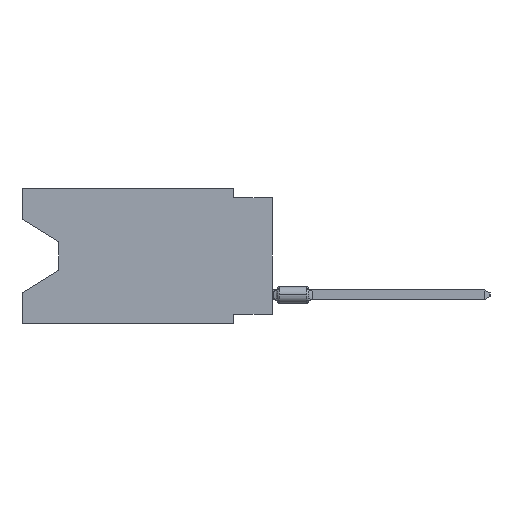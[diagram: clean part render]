
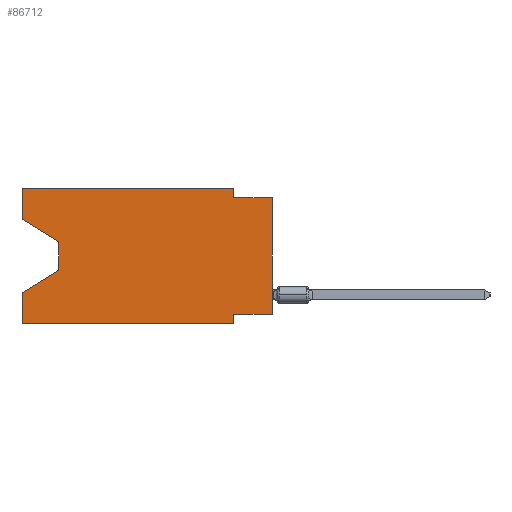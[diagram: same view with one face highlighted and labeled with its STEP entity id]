
A CAD part, left-side view. The second image highlights one B-rep face of the part: STEP entity #86712.
In plain terms, the highlighted planar face has unit normal (-1, 0, 0).
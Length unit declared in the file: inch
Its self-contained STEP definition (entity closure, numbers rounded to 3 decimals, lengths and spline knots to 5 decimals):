
#59 = DIRECTION ( 'NONE',  ( 0., 0., -1. ) ) ;
#190 = EDGE_CURVE ( 'NONE', #42665, #22390, #9721, .T. ) ;
#975 = DIRECTION ( 'NONE',  ( 0., -1., 0. ) ) ;
#1754 = DIRECTION ( 'NONE',  ( 0., 0., -1. ) ) ;
#4602 = VERTEX_POINT ( 'NONE', #24832 ) ;
#4651 = DIRECTION ( 'NONE',  ( 0., 0., 1. ) ) ;
#4712 = LINE ( 'NONE', #54291, #21248 ) ;
#5526 = EDGE_CURVE ( 'NONE', #4602, #62011, #58702, .T. ) ;
#5582 = LINE ( 'NONE', #12265, #63702 ) ;
#7689 = ORIENTED_EDGE ( 'NONE', *, *, #39928, .T. ) ;
#7878 = EDGE_LOOP ( 'NONE', ( #89855, #53086, #50535, #82369, #21418, #40404, #60067, #7689, #98472, #72064, #13869, #52340 ) ) ;
#8539 = CARTESIAN_POINT ( 'NONE',  ( 0., 0.645, -0.08025 ) ) ;
#9721 = LINE ( 'NONE', #57287, #65462 ) ;
#10214 = DIRECTION ( 'NONE',  ( 0., 0., 1. ) ) ;
#10752 = CARTESIAN_POINT ( 'NONE',  ( 0., 0.645, -0.08025 ) ) ;
#11148 = VECTOR ( 'NONE', #1754, 39.37008 ) ;
#11389 = EDGE_CURVE ( 'NONE', #88643, #62011, #37881, .T. ) ;
#12265 = CARTESIAN_POINT ( 'NONE',  ( 0., 0.645, -0.35 ) ) ;
#13869 = ORIENTED_EDGE ( 'NONE', *, *, #35759, .F. ) ;
#16514 = CARTESIAN_POINT ( 'NONE',  ( 0., 0., -0.325 ) ) ;
#16777 = VECTOR ( 'NONE', #67468, 39.37008 ) ;
#16951 = CARTESIAN_POINT ( 'NONE',  ( 0., 0., -0.025 ) ) ;
#17165 = CARTESIAN_POINT ( 'NONE',  ( 0., 0.55, -0.138 ) ) ;
#18615 = DIRECTION ( 'NONE',  ( 0., -1., 0. ) ) ;
#19096 = DIRECTION ( 'NONE',  ( 0., 0., -1. ) ) ;
#20589 = PLANE ( 'NONE',  #83614 ) ;
#21248 = VECTOR ( 'NONE', #59, 39.37008 ) ;
#21418 = ORIENTED_EDGE ( 'NONE', *, *, #82533, .T. ) ;
#22390 = VERTEX_POINT ( 'NONE', #92120 ) ;
#22966 = CARTESIAN_POINT ( 'NONE',  ( 0., 0.645, -0.35 ) ) ;
#23075 = VERTEX_POINT ( 'NONE', #59653 ) ;
#23922 = VECTOR ( 'NONE', #71784, 39.37008 ) ;
#24470 = VECTOR ( 'NONE', #4651, 39.37008 ) ;
#24832 = CARTESIAN_POINT ( 'NONE',  ( 0., 0.55, -0.212 ) ) ;
#26291 = CARTESIAN_POINT ( 'NONE',  ( 0., 0., -0.025 ) ) ;
#26933 = EDGE_CURVE ( 'NONE', #29453, #23075, #73314, .T. ) ;
#28447 = CARTESIAN_POINT ( 'NONE',  ( 0., 0.645, -0.26975 ) ) ;
#29453 = VERTEX_POINT ( 'NONE', #84369 ) ;
#29799 = CARTESIAN_POINT ( 'NONE',  ( 0., 0.1, -0.325 ) ) ;
#32194 = VECTOR ( 'NONE', #39957, 39.37008 ) ;
#32704 = CARTESIAN_POINT ( 'NONE',  ( 0., 0.645, 0. ) ) ;
#32901 = VECTOR ( 'NONE', #18615, 39.37008 ) ;
#35759 = EDGE_CURVE ( 'NONE', #22390, #29453, #57224, .T. ) ;
#35779 = VECTOR ( 'NONE', #975, 39.37008 ) ;
#37041 = EDGE_CURVE ( 'NONE', #49815, #4602, #4712, .T. ) ;
#37881 = LINE ( 'NONE', #100285, #24470 ) ;
#38075 = VERTEX_POINT ( 'NONE', #58628 ) ;
#39928 = EDGE_CURVE ( 'NONE', #38075, #73251, #99680, .T. ) ;
#39957 = DIRECTION ( 'NONE',  ( 0., -0.855, -0.519 ) ) ;
#40404 = ORIENTED_EDGE ( 'NONE', *, *, #52274, .F. ) ;
#42665 = VERTEX_POINT ( 'NONE', #8539 ) ;
#48315 = CARTESIAN_POINT ( 'NONE',  ( 0., 0.1, -0.35 ) ) ;
#49815 = VERTEX_POINT ( 'NONE', #17165 ) ;
#50284 = DIRECTION ( 'NONE',  ( 0., 0., -1. ) ) ;
#50535 = ORIENTED_EDGE ( 'NONE', *, *, #5526, .T. ) ;
#50595 = EDGE_CURVE ( 'NONE', #42665, #49815, #80851, .T. ) ;
#50674 = DIRECTION ( 'NONE',  ( 0., -1., 0. ) ) ;
#51620 = VECTOR ( 'NONE', #50284, 39.37008 ) ;
#52007 = CARTESIAN_POINT ( 'NONE',  ( 0., 0.1, -0.35 ) ) ;
#52274 = EDGE_CURVE ( 'NONE', #75323, #95574, #87187, .T. ) ;
#52340 = ORIENTED_EDGE ( 'NONE', *, *, #190, .F. ) ;
#53086 = ORIENTED_EDGE ( 'NONE', *, *, #37041, .T. ) ;
#54291 = CARTESIAN_POINT ( 'NONE',  ( 0., 0.55, -0.138 ) ) ;
#55984 = EDGE_CURVE ( 'NONE', #38075, #75323, #94309, .T. ) ;
#57224 = LINE ( 'NONE', #32704, #35779 ) ;
#57287 = CARTESIAN_POINT ( 'NONE',  ( 0., 0.645, 0. ) ) ;
#58505 = LINE ( 'NONE', #26291, #32901 ) ;
#58628 = CARTESIAN_POINT ( 'NONE',  ( 0., 0., -0.325 ) ) ;
#58702 = LINE ( 'NONE', #67383, #63312 ) ;
#59653 = CARTESIAN_POINT ( 'NONE',  ( 0., 0.1, -0.025 ) ) ;
#60067 = ORIENTED_EDGE ( 'NONE', *, *, #55984, .F. ) ;
#62011 = VERTEX_POINT ( 'NONE', #28447 ) ;
#63312 = VECTOR ( 'NONE', #66896, 39.37008 ) ;
#63702 = VECTOR ( 'NONE', #50674, 39.37008 ) ;
#65462 = VECTOR ( 'NONE', #10214, 39.37008 ) ;
#66896 = DIRECTION ( 'NONE',  ( 0., 0.855, -0.519 ) ) ;
#67383 = CARTESIAN_POINT ( 'NONE',  ( 0., 0.55, -0.212 ) ) ;
#67468 = DIRECTION ( 'NONE',  ( 0., 0., 1. ) ) ;
#71784 = DIRECTION ( 'NONE',  ( 0., 1., 0. ) ) ;
#72064 = ORIENTED_EDGE ( 'NONE', *, *, #26933, .F. ) ;
#72127 = EDGE_CURVE ( 'NONE', #23075, #73251, #58505, .T. ) ;
#73251 = VERTEX_POINT ( 'NONE', #16951 ) ;
#73314 = LINE ( 'NONE', #91168, #51620 ) ;
#75323 = VERTEX_POINT ( 'NONE', #29799 ) ;
#80851 = LINE ( 'NONE', #10752, #32194 ) ;
#82369 = ORIENTED_EDGE ( 'NONE', *, *, #11389, .F. ) ;
#82479 = CARTESIAN_POINT ( 'NONE',  ( 0., 0.645, 0. ) ) ;
#82533 = EDGE_CURVE ( 'NONE', #88643, #95574, #5582, .T. ) ;
#83614 = AXIS2_PLACEMENT_3D ( 'NONE', #82479, #89176, #19096 ) ;
#84369 = CARTESIAN_POINT ( 'NONE',  ( 0., 0.1, 0. ) ) ;
#86712 = ADVANCED_FACE ( 'NONE', ( #97368 ), #20589, .F. ) ;
#87187 = LINE ( 'NONE', #48315, #11148 ) ;
#88643 = VERTEX_POINT ( 'NONE', #22966 ) ;
#89176 = DIRECTION ( 'NONE',  ( 1., 0., 0. ) ) ;
#89855 = ORIENTED_EDGE ( 'NONE', *, *, #50595, .T. ) ;
#91004 = CARTESIAN_POINT ( 'NONE',  ( 0., 0., 0. ) ) ;
#91168 = CARTESIAN_POINT ( 'NONE',  ( 0., 0.1, 0. ) ) ;
#92120 = CARTESIAN_POINT ( 'NONE',  ( 0., 0.645, 0. ) ) ;
#94309 = LINE ( 'NONE', #16514, #23922 ) ;
#95574 = VERTEX_POINT ( 'NONE', #52007 ) ;
#97368 = FACE_OUTER_BOUND ( 'NONE', #7878, .T. ) ;
#98472 = ORIENTED_EDGE ( 'NONE', *, *, #72127, .F. ) ;
#99680 = LINE ( 'NONE', #91004, #16777 ) ;
#100285 = CARTESIAN_POINT ( 'NONE',  ( 0., 0.645, 0. ) ) ;
